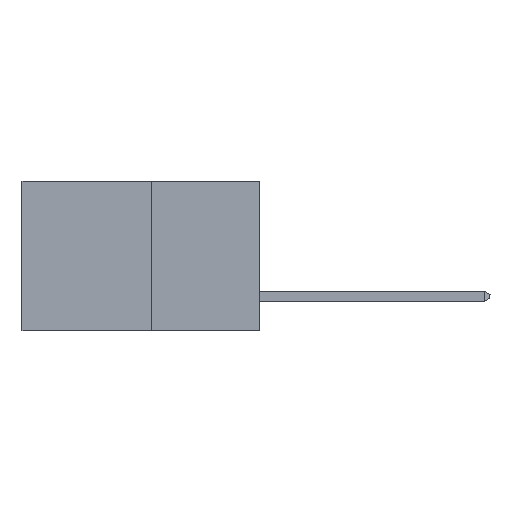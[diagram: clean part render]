
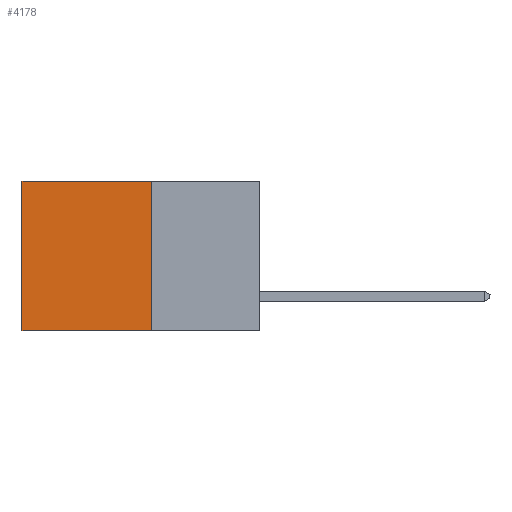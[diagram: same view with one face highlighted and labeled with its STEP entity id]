
A CAD part, left-side view. The second image highlights one B-rep face of the part: STEP entity #4178.
In plain terms, the highlighted planar face has unit normal (-1, 0, 0).
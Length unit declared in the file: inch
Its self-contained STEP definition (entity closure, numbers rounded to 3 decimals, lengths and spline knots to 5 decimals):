
#25 = ORIENTED_EDGE ( 'NONE', *, *, #3002, .T. ) ;
#109 = DIRECTION ( 'NONE',  ( 0., 0., -1. ) ) ;
#133 = DIRECTION ( 'NONE',  ( 0., 0., -1. ) ) ;
#135 = CARTESIAN_POINT ( 'NONE',  ( 0.277, 0.59, -0.37 ) ) ;
#136 = DIRECTION ( 'NONE',  ( 1., 0., 0. ) ) ;
#217 = PLANE ( 'NONE',  #8345 ) ;
#258 = CARTESIAN_POINT ( 'NONE',  ( 0.277, 0.27, -0.37 ) ) ;
#355 = CARTESIAN_POINT ( 'NONE',  ( 0.277, 0.27, 0. ) ) ;
#853 = DIRECTION ( 'NONE',  ( 0., 0., -1. ) ) ;
#931 = EDGE_LOOP ( 'NONE', ( #3658, #8409, #7324, #25 ) ) ;
#1181 = DIRECTION ( 'NONE',  ( 0., 1., 0. ) ) ;
#1234 = EDGE_CURVE ( 'NONE', #7501, #8825, #6102, .T. ) ;
#1555 = CARTESIAN_POINT ( 'NONE',  ( 0.277, 0.27, -0.37 ) ) ;
#2164 = VERTEX_POINT ( 'NONE', #9404 ) ;
#2291 = VERTEX_POINT ( 'NONE', #7627 ) ;
#3002 = EDGE_CURVE ( 'NONE', #7501, #2291, #8037, .T. ) ;
#3352 = EDGE_CURVE ( 'NONE', #2291, #2164, #8251, .T. ) ;
#3658 = ORIENTED_EDGE ( 'NONE', *, *, #3352, .T. ) ;
#3696 = CARTESIAN_POINT ( 'NONE',  ( 0.277, 0.27, -0.37 ) ) ;
#4178 = ADVANCED_FACE ( 'NONE', ( #9454 ), #217, .F. ) ;
#4647 = DIRECTION ( 'NONE',  ( 0., 1., 0. ) ) ;
#4692 = CARTESIAN_POINT ( 'NONE',  ( 0.277, 0.27, 0. ) ) ;
#5962 = EDGE_CURVE ( 'NONE', #8825, #2164, #9564, .T. ) ;
#6102 = LINE ( 'NONE', #1555, #9319 ) ;
#6423 = VECTOR ( 'NONE', #4647, 39.37008 ) ;
#6449 = CARTESIAN_POINT ( 'NONE',  ( 0.277, 0.27, -0.37 ) ) ;
#7324 = ORIENTED_EDGE ( 'NONE', *, *, #1234, .F. ) ;
#7501 = VERTEX_POINT ( 'NONE', #355 ) ;
#7627 = CARTESIAN_POINT ( 'NONE',  ( 0.277, 0.59, 0. ) ) ;
#8019 = VECTOR ( 'NONE', #1181, 39.37008 ) ;
#8025 = VECTOR ( 'NONE', #109, 39.37008 ) ;
#8037 = LINE ( 'NONE', #4692, #6423 ) ;
#8251 = LINE ( 'NONE', #135, #8025 ) ;
#8345 = AXIS2_PLACEMENT_3D ( 'NONE', #258, #136, #133 ) ;
#8409 = ORIENTED_EDGE ( 'NONE', *, *, #5962, .F. ) ;
#8825 = VERTEX_POINT ( 'NONE', #6449 ) ;
#9319 = VECTOR ( 'NONE', #853, 39.37008 ) ;
#9404 = CARTESIAN_POINT ( 'NONE',  ( 0.277, 0.59, -0.37 ) ) ;
#9454 = FACE_OUTER_BOUND ( 'NONE', #931, .T. ) ;
#9564 = LINE ( 'NONE', #3696, #8019 ) ;
